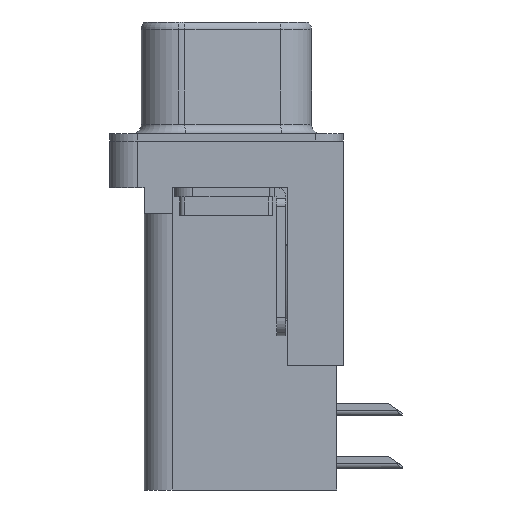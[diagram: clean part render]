
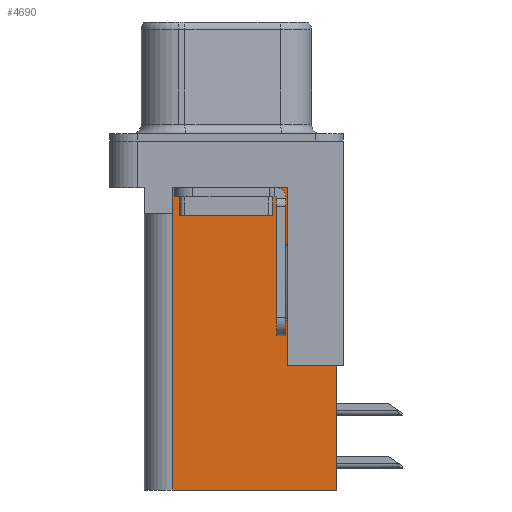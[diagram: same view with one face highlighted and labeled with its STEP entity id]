
A CAD part, left-side view. The second image highlights one B-rep face of the part: STEP entity #4690.
In plain terms, the highlighted planar face has unit normal (-1, 0, 0).
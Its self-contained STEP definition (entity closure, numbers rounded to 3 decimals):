
#313 = VECTOR ( 'NONE', #2846, 1000. ) ;
#506 = DIRECTION ( 'NONE',  ( 0., 1., 0. ) ) ;
#521 = EDGE_CURVE ( 'NONE', #4613, #12875, #9822, .T. ) ;
#1089 = CARTESIAN_POINT ( 'NONE',  ( 3.765, -3.295, -2.5 ) ) ;
#1451 = PLANE ( 'NONE',  #17665 ) ;
#1681 = CARTESIAN_POINT ( 'NONE',  ( 3.765, 2.895, -2.5 ) ) ;
#2220 = VECTOR ( 'NONE', #506, 1000. ) ;
#2846 = DIRECTION ( 'NONE',  ( 0., 0., 1. ) ) ;
#3761 = VECTOR ( 'NONE', #20393, 1000. ) ;
#4070 = VECTOR ( 'NONE', #9460, 1000. ) ;
#4270 = CARTESIAN_POINT ( 'NONE',  ( 3.765, 2.895, -3.9 ) ) ;
#4390 = DIRECTION ( 'NONE',  ( 0., 1., 0. ) ) ;
#4407 = DIRECTION ( 'NONE',  ( 1., 0., 0. ) ) ;
#4479 = DIRECTION ( 'NONE',  ( 0., 1., 0. ) ) ;
#4569 = VECTOR ( 'NONE', #12390, 1000. ) ;
#4613 = VERTEX_POINT ( 'NONE', #1089 ) ;
#4683 = ORIENTED_EDGE ( 'NONE', *, *, #9287, .F. ) ;
#4690 = ADVANCED_FACE ( 'NONE', ( #12474 ), #1451, .F. ) ;
#5143 = LINE ( 'NONE', #12473, #313 ) ;
#5476 = CARTESIAN_POINT ( 'NONE',  ( 3.765, -5.925, -12.05 ) ) ;
#5848 = CARTESIAN_POINT ( 'NONE',  ( 3.765, 0., -3.9 ) ) ;
#5984 = VECTOR ( 'NONE', #15993, 1000. ) ;
#7123 = LINE ( 'NONE', #11703, #2220 ) ;
#7910 = CARTESIAN_POINT ( 'NONE',  ( 3.765, 2.895, -3.9 ) ) ;
#7946 = ORIENTED_EDGE ( 'NONE', *, *, #521, .T. ) ;
#8468 = LINE ( 'NONE', #9302, #11598 ) ;
#8775 = VERTEX_POINT ( 'NONE', #20346 ) ;
#9048 = CARTESIAN_POINT ( 'NONE',  ( 3.765, -3.295, -18.76 ) ) ;
#9146 = VERTEX_POINT ( 'NONE', #5476 ) ;
#9287 = EDGE_CURVE ( 'NONE', #17449, #10558, #5143, .T. ) ;
#9302 = CARTESIAN_POINT ( 'NONE',  ( 3.765, -3.295, -18.76 ) ) ;
#9460 = DIRECTION ( 'NONE',  ( 0., 0., -1. ) ) ;
#9822 = LINE ( 'NONE', #14525, #17905 ) ;
#10342 = CARTESIAN_POINT ( 'NONE',  ( 3.765, 2.925, -18.76 ) ) ;
#10558 = VERTEX_POINT ( 'NONE', #19750 ) ;
#10787 = CARTESIAN_POINT ( 'NONE',  ( 3.765, -5.925, -2. ) ) ;
#11198 = EDGE_CURVE ( 'NONE', #9146, #18773, #7123, .T. ) ;
#11430 = ORIENTED_EDGE ( 'NONE', *, *, #16199, .F. ) ;
#11598 = VECTOR ( 'NONE', #15646, 1000. ) ;
#11703 = CARTESIAN_POINT ( 'NONE',  ( 3.765, -6.295, -12.05 ) ) ;
#12147 = EDGE_CURVE ( 'NONE', #8775, #17449, #18302, .T. ) ;
#12390 = DIRECTION ( 'NONE',  ( 0., 0., -1. ) ) ;
#12473 = CARTESIAN_POINT ( 'NONE',  ( 3.765, 2.925, -18.76 ) ) ;
#12474 = FACE_OUTER_BOUND ( 'NONE', #14473, .T. ) ;
#12875 = VERTEX_POINT ( 'NONE', #1681 ) ;
#14114 = EDGE_CURVE ( 'NONE', #18773, #4613, #8468, .T. ) ;
#14473 = EDGE_LOOP ( 'NONE', ( #7946, #15377, #17684, #4683, #16372, #11430, #19001, #19560 ) ) ;
#14525 = CARTESIAN_POINT ( 'NONE',  ( 3.765, -3.295, -2.5 ) ) ;
#15377 = ORIENTED_EDGE ( 'NONE', *, *, #15648, .T. ) ;
#15646 = DIRECTION ( 'NONE',  ( 0., 0., 1. ) ) ;
#15648 = EDGE_CURVE ( 'NONE', #12875, #20441, #17952, .T. ) ;
#15993 = DIRECTION ( 'NONE',  ( 0., 1., 0. ) ) ;
#16199 = EDGE_CURVE ( 'NONE', #9146, #8775, #17929, .T. ) ;
#16372 = ORIENTED_EDGE ( 'NONE', *, *, #12147, .F. ) ;
#16400 = CARTESIAN_POINT ( 'NONE',  ( 3.765, -3.295, -12.05 ) ) ;
#16586 = LINE ( 'NONE', #5848, #3761 ) ;
#17449 = VERTEX_POINT ( 'NONE', #10342 ) ;
#17571 = EDGE_CURVE ( 'NONE', #20441, #10558, #16586, .T. ) ;
#17665 = AXIS2_PLACEMENT_3D ( 'NONE', #9048, #4407, #4479 ) ;
#17684 = ORIENTED_EDGE ( 'NONE', *, *, #17571, .T. ) ;
#17905 = VECTOR ( 'NONE', #4390, 1000. ) ;
#17929 = LINE ( 'NONE', #10787, #4569 ) ;
#17952 = LINE ( 'NONE', #7910, #4070 ) ;
#18302 = LINE ( 'NONE', #20916, #5984 ) ;
#18773 = VERTEX_POINT ( 'NONE', #16400 ) ;
#19001 = ORIENTED_EDGE ( 'NONE', *, *, #11198, .T. ) ;
#19560 = ORIENTED_EDGE ( 'NONE', *, *, #14114, .T. ) ;
#19750 = CARTESIAN_POINT ( 'NONE',  ( 3.765, 2.925, -3.9 ) ) ;
#20346 = CARTESIAN_POINT ( 'NONE',  ( 3.765, -5.925, -18.76 ) ) ;
#20393 = DIRECTION ( 'NONE',  ( 0., 1., 0. ) ) ;
#20441 = VERTEX_POINT ( 'NONE', #4270 ) ;
#20916 = CARTESIAN_POINT ( 'NONE',  ( 3.765, -3.295, -18.76 ) ) ;
